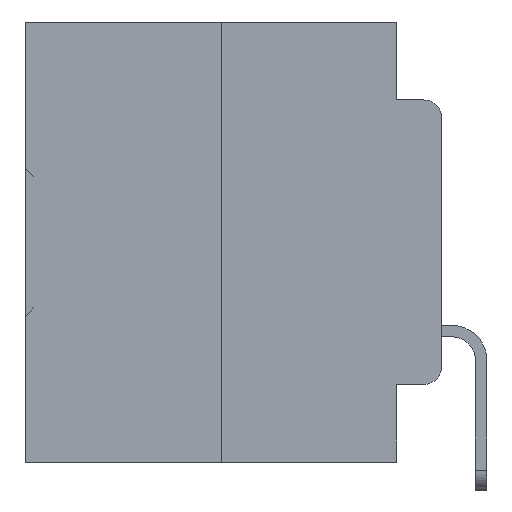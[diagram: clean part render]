
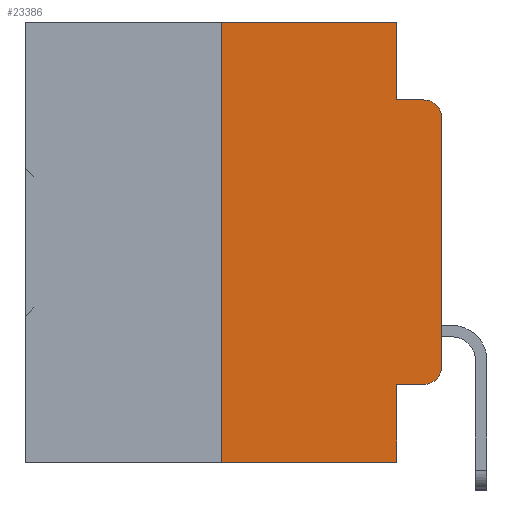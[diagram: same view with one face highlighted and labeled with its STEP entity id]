
A CAD part, left-side view. The second image highlights one B-rep face of the part: STEP entity #23386.
In plain terms, the highlighted planar face has unit normal (-1, 0, 0).
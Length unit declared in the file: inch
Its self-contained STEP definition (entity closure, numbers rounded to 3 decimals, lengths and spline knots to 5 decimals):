
#477 = LINE ( 'NONE', #19853, #15977 ) ;
#515 = EDGE_CURVE ( 'NONE', #36590, #15202, #11417, .T. ) ;
#566 = VERTEX_POINT ( 'NONE', #32649 ) ;
#1425 = LINE ( 'NONE', #12543, #31069 ) ;
#2315 = VERTEX_POINT ( 'NONE', #26336 ) ;
#2760 = CARTESIAN_POINT ( 'NONE',  ( 0., 0.051, -0.4115 ) ) ;
#2801 = VERTEX_POINT ( 'NONE', #10648 ) ;
#3750 = FACE_OUTER_BOUND ( 'NONE', #25722, .T. ) ;
#3757 = EDGE_CURVE ( 'NONE', #13117, #2801, #7101, .T. ) ;
#4100 = ORIENTED_EDGE ( 'NONE', *, *, #14257, .T. ) ;
#5530 = DIRECTION ( 'NONE',  ( 0., 0., -1. ) ) ;
#6155 = CARTESIAN_POINT ( 'NONE',  ( 0., 0.051, 0. ) ) ;
#6456 = AXIS2_PLACEMENT_3D ( 'NONE', #30639, #13680, #33491 ) ;
#6496 = EDGE_CURVE ( 'NONE', #21877, #15202, #34401, .T. ) ;
#6842 = PLANE ( 'NONE',  #25570 ) ;
#7101 = LINE ( 'NONE', #14863, #21406 ) ;
#8399 = VECTOR ( 'NONE', #27074, 39.37008 ) ;
#9651 = CARTESIAN_POINT ( 'NONE',  ( 0., 0.473, 0. ) ) ;
#9768 = DIRECTION ( 'NONE',  ( 0., 0., -1. ) ) ;
#10009 = CARTESIAN_POINT ( 'NONE',  ( 0., 0.25, -0.5 ) ) ;
#10139 = EDGE_CURVE ( 'NONE', #13117, #34504, #1425, .T. ) ;
#10648 = CARTESIAN_POINT ( 'NONE',  ( 0., 0.25, 0. ) ) ;
#11417 = LINE ( 'NONE', #26046, #12296 ) ;
#11525 = ORIENTED_EDGE ( 'NONE', *, *, #17370, .F. ) ;
#11847 = CARTESIAN_POINT ( 'NONE',  ( 0., 0.051, -0.0885 ) ) ;
#12296 = VECTOR ( 'NONE', #34829, 39.37008 ) ;
#12479 = DIRECTION ( 'NONE',  ( -1., 0., 0. ) ) ;
#12543 = CARTESIAN_POINT ( 'NONE',  ( 0., 0.473, -0.5 ) ) ;
#12621 = VECTOR ( 'NONE', #34717, 39.37008 ) ;
#13117 = VERTEX_POINT ( 'NONE', #10009 ) ;
#13291 = ORIENTED_EDGE ( 'NONE', *, *, #15217, .T. ) ;
#13680 = DIRECTION ( 'NONE',  ( -1., 0., 0. ) ) ;
#13726 = ORIENTED_EDGE ( 'NONE', *, *, #3757, .F. ) ;
#13812 = LINE ( 'NONE', #17230, #35463 ) ;
#13863 = CARTESIAN_POINT ( 'NONE',  ( 0., 0.051, -0.5 ) ) ;
#14257 = EDGE_CURVE ( 'NONE', #566, #21877, #20184, .T. ) ;
#14863 = CARTESIAN_POINT ( 'NONE',  ( 0., 0.25, 0. ) ) ;
#15202 = VERTEX_POINT ( 'NONE', #36741 ) ;
#15217 = EDGE_CURVE ( 'NONE', #2315, #27989, #23186, .T. ) ;
#15705 = EDGE_CURVE ( 'NONE', #27989, #566, #28028, .T. ) ;
#15966 = ORIENTED_EDGE ( 'NONE', *, *, #15705, .T. ) ;
#15977 = VECTOR ( 'NONE', #5530, 39.37008 ) ;
#16405 = ORIENTED_EDGE ( 'NONE', *, *, #10139, .T. ) ;
#16897 = LINE ( 'NONE', #35441, #8399 ) ;
#17230 = CARTESIAN_POINT ( 'NONE',  ( 0., 0.473, 0. ) ) ;
#17370 = EDGE_CURVE ( 'NONE', #2315, #34504, #16897, .T. ) ;
#17725 = ORIENTED_EDGE ( 'NONE', *, *, #22519, .F. ) ;
#19853 = CARTESIAN_POINT ( 'NONE',  ( 0., 0.051, 0. ) ) ;
#20038 = DIRECTION ( 'NONE',  ( 0., -1., 0. ) ) ;
#20046 = DIRECTION ( 'NONE',  ( 0., -1., 0. ) ) ;
#20184 = LINE ( 'NONE', #29030, #12621 ) ;
#21097 = DIRECTION ( 'NONE',  ( 0., -1., 0. ) ) ;
#21226 = ORIENTED_EDGE ( 'NONE', *, *, #6496, .T. ) ;
#21406 = VECTOR ( 'NONE', #27467, 39.37008 ) ;
#21877 = VERTEX_POINT ( 'NONE', #23310 ) ;
#22519 = EDGE_CURVE ( 'NONE', #2801, #28339, #13812, .T. ) ;
#23014 = ORIENTED_EDGE ( 'NONE', *, *, #515, .F. ) ;
#23186 = LINE ( 'NONE', #2760, #30717 ) ;
#23310 = CARTESIAN_POINT ( 'NONE',  ( 0., 0., -0.1085 ) ) ;
#23386 = ADVANCED_FACE ( 'NONE', ( #3750 ), #6842, .F. ) ;
#23478 = AXIS2_PLACEMENT_3D ( 'NONE', #29448, #12479, #32280 ) ;
#23718 = EDGE_CURVE ( 'NONE', #28339, #36590, #477, .T. ) ;
#25570 = AXIS2_PLACEMENT_3D ( 'NONE', #9651, #26797, #9768 ) ;
#25722 = EDGE_LOOP ( 'NONE', ( #4100, #21226, #23014, #30095, #17725, #13726, #16405, #11525, #13291, #15966 ) ) ;
#26046 = CARTESIAN_POINT ( 'NONE',  ( 0., 0.051, -0.0885 ) ) ;
#26336 = CARTESIAN_POINT ( 'NONE',  ( 0., 0.051, -0.4115 ) ) ;
#26797 = DIRECTION ( 'NONE',  ( 1., 0., 0. ) ) ;
#27074 = DIRECTION ( 'NONE',  ( 0., 0., -1. ) ) ;
#27467 = DIRECTION ( 'NONE',  ( 0., 0., 1. ) ) ;
#27989 = VERTEX_POINT ( 'NONE', #30381 ) ;
#28028 = CIRCLE ( 'NONE', #6456, 0.02 ) ;
#28339 = VERTEX_POINT ( 'NONE', #6155 ) ;
#29030 = CARTESIAN_POINT ( 'NONE',  ( 0., 0., 0. ) ) ;
#29448 = CARTESIAN_POINT ( 'NONE',  ( 0., 0.02, -0.1085 ) ) ;
#30095 = ORIENTED_EDGE ( 'NONE', *, *, #23718, .F. ) ;
#30381 = CARTESIAN_POINT ( 'NONE',  ( 0., 0.02, -0.4115 ) ) ;
#30639 = CARTESIAN_POINT ( 'NONE',  ( 0., 0.02, -0.3915 ) ) ;
#30717 = VECTOR ( 'NONE', #20038, 39.37008 ) ;
#31069 = VECTOR ( 'NONE', #21097, 39.37008 ) ;
#32280 = DIRECTION ( 'NONE',  ( 0., 0., -1. ) ) ;
#32649 = CARTESIAN_POINT ( 'NONE',  ( 0., 0., -0.3915 ) ) ;
#33491 = DIRECTION ( 'NONE',  ( 0., 0., -1. ) ) ;
#34401 = CIRCLE ( 'NONE', #23478, 0.02 ) ;
#34504 = VERTEX_POINT ( 'NONE', #13863 ) ;
#34717 = DIRECTION ( 'NONE',  ( 0., 0., 1. ) ) ;
#34829 = DIRECTION ( 'NONE',  ( 0., -1., 0. ) ) ;
#35441 = CARTESIAN_POINT ( 'NONE',  ( 0., 0.051, 0. ) ) ;
#35463 = VECTOR ( 'NONE', #20046, 39.37008 ) ;
#36590 = VERTEX_POINT ( 'NONE', #11847 ) ;
#36741 = CARTESIAN_POINT ( 'NONE',  ( 0., 0.02, -0.0885 ) ) ;
